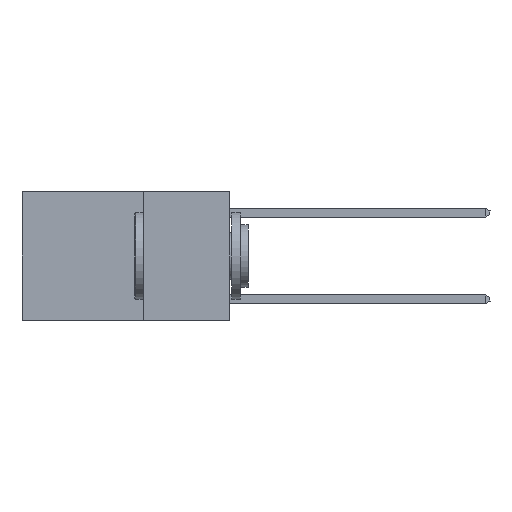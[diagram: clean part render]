
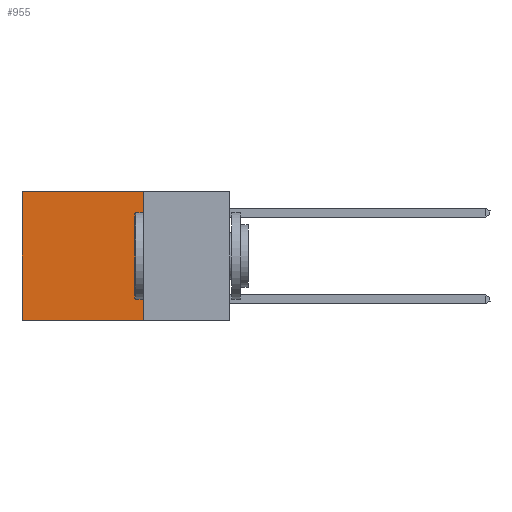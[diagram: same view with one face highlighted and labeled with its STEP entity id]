
A CAD part, left-side view. The second image highlights one B-rep face of the part: STEP entity #955.
In plain terms, the highlighted planar face has unit normal (-1, 0, 0).
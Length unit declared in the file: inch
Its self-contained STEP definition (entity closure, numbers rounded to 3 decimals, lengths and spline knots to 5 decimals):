
#598 = EDGE_CURVE ( 'NONE', #8069, #3591, #3043, .T. ) ;
#662 = CARTESIAN_POINT ( 'NONE',  ( 0.2625, 0.6, -0.37 ) ) ;
#955 = ADVANCED_FACE ( 'NONE', ( #5825 ), #13891, .F. ) ;
#1482 = CARTESIAN_POINT ( 'NONE',  ( 0.2625, 0.25, 0. ) ) ;
#1603 = CARTESIAN_POINT ( 'NONE',  ( 0.2625, 0.25, 0. ) ) ;
#2628 = CARTESIAN_POINT ( 'NONE',  ( 0.2625, 0.6, 0. ) ) ;
#2863 = LINE ( 'NONE', #5790, #3866 ) ;
#3043 = LINE ( 'NONE', #15775, #16284 ) ;
#3591 = VERTEX_POINT ( 'NONE', #8092 ) ;
#3866 = VECTOR ( 'NONE', #12033, 39.37008 ) ;
#4096 = ORIENTED_EDGE ( 'NONE', *, *, #4177, .T. ) ;
#4177 = EDGE_CURVE ( 'NONE', #12148, #13081, #2863, .T. ) ;
#4355 = EDGE_LOOP ( 'NONE', ( #4096, #14482, #13457, #15782 ) ) ;
#4805 = DIRECTION ( 'NONE',  ( 0., 0., -1. ) ) ;
#5148 = DIRECTION ( 'NONE',  ( 0., 1., 0. ) ) ;
#5790 = CARTESIAN_POINT ( 'NONE',  ( 0.2625, 0.6, 0. ) ) ;
#5825 = FACE_OUTER_BOUND ( 'NONE', #4355, .T. ) ;
#6212 = DIRECTION ( 'NONE',  ( 1., 0., 0. ) ) ;
#8069 = VERTEX_POINT ( 'NONE', #1482 ) ;
#8092 = CARTESIAN_POINT ( 'NONE',  ( 0.2625, 0.25, -0.37 ) ) ;
#8270 = DIRECTION ( 'NONE',  ( 0., 0., -1. ) ) ;
#8636 = CARTESIAN_POINT ( 'NONE',  ( 0.2625, 0.25, 0. ) ) ;
#8958 = EDGE_CURVE ( 'NONE', #8069, #12148, #14299, .T. ) ;
#9345 = AXIS2_PLACEMENT_3D ( 'NONE', #8636, #6212, #4805 ) ;
#9420 = VECTOR ( 'NONE', #5148, 39.37008 ) ;
#10559 = DIRECTION ( 'NONE',  ( 0., 1., 0. ) ) ;
#11914 = VECTOR ( 'NONE', #10559, 39.37008 ) ;
#12033 = DIRECTION ( 'NONE',  ( 0., 0., -1. ) ) ;
#12148 = VERTEX_POINT ( 'NONE', #2628 ) ;
#12915 = CARTESIAN_POINT ( 'NONE',  ( 0.2625, 0.25, -0.37 ) ) ;
#13081 = VERTEX_POINT ( 'NONE', #662 ) ;
#13457 = ORIENTED_EDGE ( 'NONE', *, *, #598, .F. ) ;
#13891 = PLANE ( 'NONE',  #9345 ) ;
#14299 = LINE ( 'NONE', #1603, #11914 ) ;
#14482 = ORIENTED_EDGE ( 'NONE', *, *, #15449, .F. ) ;
#15449 = EDGE_CURVE ( 'NONE', #3591, #13081, #16237, .T. ) ;
#15775 = CARTESIAN_POINT ( 'NONE',  ( 0.2625, 0.25, 0. ) ) ;
#15782 = ORIENTED_EDGE ( 'NONE', *, *, #8958, .T. ) ;
#16237 = LINE ( 'NONE', #12915, #9420 ) ;
#16284 = VECTOR ( 'NONE', #8270, 39.37008 ) ;
